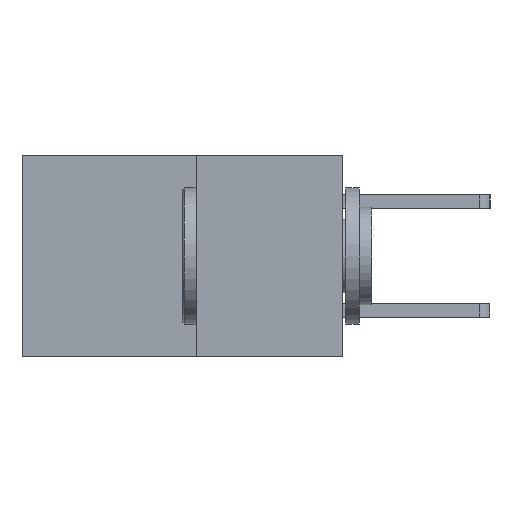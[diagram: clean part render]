
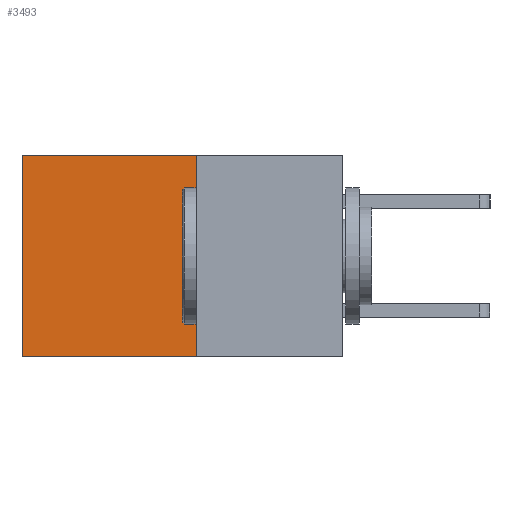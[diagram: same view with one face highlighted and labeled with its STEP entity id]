
A CAD part, left-side view. The second image highlights one B-rep face of the part: STEP entity #3493.
In plain terms, the highlighted planar face has unit normal (-1, 0, 0).
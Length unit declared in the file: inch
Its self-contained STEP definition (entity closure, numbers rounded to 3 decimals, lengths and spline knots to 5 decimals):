
#851 = EDGE_CURVE ( 'NONE', #3560, #7684, #2532, .T. ) ;
#1140 = DIRECTION ( 'NONE',  ( 0., 1., 0. ) ) ;
#1180 = VECTOR ( 'NONE', #1140, 39.37008 ) ;
#1231 = ORIENTED_EDGE ( 'NONE', *, *, #4555, .F. ) ;
#1235 = CARTESIAN_POINT ( 'NONE',  ( 0.277, 0.27, -0.37 ) ) ;
#1770 = CARTESIAN_POINT ( 'NONE',  ( 0.277, 0.27, 0. ) ) ;
#2412 = DIRECTION ( 'NONE',  ( 0., 1., 0. ) ) ;
#2532 = LINE ( 'NONE', #5521, #4498 ) ;
#2845 = LINE ( 'NONE', #7511, #3126 ) ;
#3126 = VECTOR ( 'NONE', #2412, 39.37008 ) ;
#3492 = CARTESIAN_POINT ( 'NONE',  ( 0.277, 0.27, -0.37 ) ) ;
#3493 = ADVANCED_FACE ( 'NONE', ( #9103 ), #5747, .F. ) ;
#3536 = LINE ( 'NONE', #1235, #1180 ) ;
#3560 = VERTEX_POINT ( 'NONE', #1770 ) ;
#3592 = ORIENTED_EDGE ( 'NONE', *, *, #851, .F. ) ;
#4316 = AXIS2_PLACEMENT_3D ( 'NONE', #6654, #5680, #5635 ) ;
#4498 = VECTOR ( 'NONE', #9162, 39.37008 ) ;
#4555 = EDGE_CURVE ( 'NONE', #7684, #6420, #3536, .T. ) ;
#5334 = VERTEX_POINT ( 'NONE', #6372 ) ;
#5521 = CARTESIAN_POINT ( 'NONE',  ( 0.277, 0.27, -0.37 ) ) ;
#5635 = DIRECTION ( 'NONE',  ( 0., 0., -1. ) ) ;
#5680 = DIRECTION ( 'NONE',  ( 1., 0., 0. ) ) ;
#5747 = PLANE ( 'NONE',  #4316 ) ;
#5824 = ORIENTED_EDGE ( 'NONE', *, *, #6177, .T. ) ;
#6177 = EDGE_CURVE ( 'NONE', #3560, #5334, #2845, .T. ) ;
#6372 = CARTESIAN_POINT ( 'NONE',  ( 0.277, 0.59, 0. ) ) ;
#6420 = VERTEX_POINT ( 'NONE', #9422 ) ;
#6654 = CARTESIAN_POINT ( 'NONE',  ( 0.277, 0.27, -0.37 ) ) ;
#7511 = CARTESIAN_POINT ( 'NONE',  ( 0.277, 0.27, 0. ) ) ;
#7684 = VERTEX_POINT ( 'NONE', #3492 ) ;
#7871 = ORIENTED_EDGE ( 'NONE', *, *, #9530, .T. ) ;
#8203 = CARTESIAN_POINT ( 'NONE',  ( 0.277, 0.59, -0.37 ) ) ;
#8342 = VECTOR ( 'NONE', #9020, 39.37008 ) ;
#8598 = LINE ( 'NONE', #8203, #8342 ) ;
#9020 = DIRECTION ( 'NONE',  ( 0., 0., -1. ) ) ;
#9103 = FACE_OUTER_BOUND ( 'NONE', #10215, .T. ) ;
#9162 = DIRECTION ( 'NONE',  ( 0., 0., -1. ) ) ;
#9422 = CARTESIAN_POINT ( 'NONE',  ( 0.277, 0.59, -0.37 ) ) ;
#9530 = EDGE_CURVE ( 'NONE', #5334, #6420, #8598, .T. ) ;
#10215 = EDGE_LOOP ( 'NONE', ( #7871, #1231, #3592, #5824 ) ) ;
